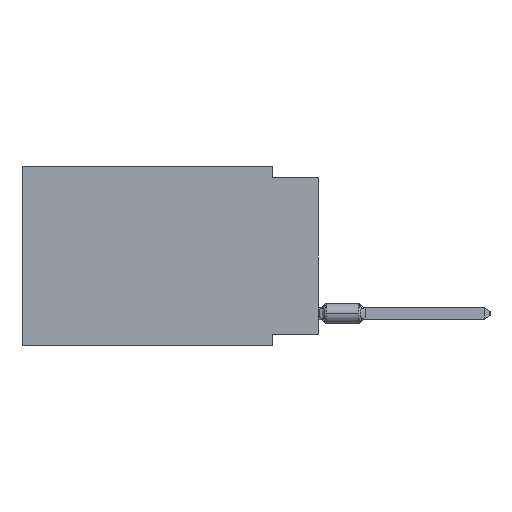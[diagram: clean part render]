
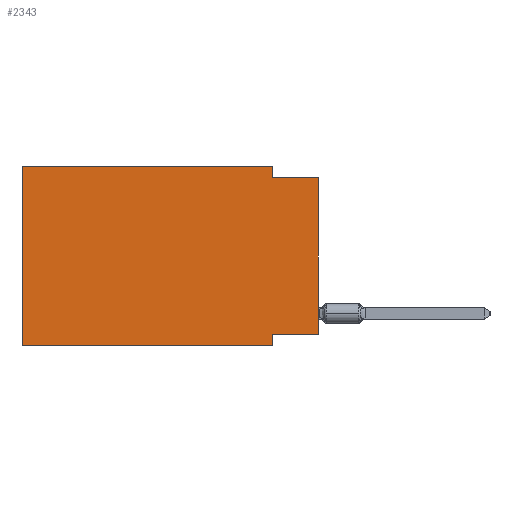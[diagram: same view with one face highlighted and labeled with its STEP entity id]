
A CAD part, left-side view. The second image highlights one B-rep face of the part: STEP entity #2343.
In plain terms, the highlighted planar face has unit normal (-1, 0, 0).
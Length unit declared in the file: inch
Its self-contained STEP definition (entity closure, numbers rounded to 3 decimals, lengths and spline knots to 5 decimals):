
#295 = CARTESIAN_POINT ( 'NONE',  ( 0., 0.1, 0. ) ) ;
#1831 = VERTEX_POINT ( 'NONE', #42576 ) ;
#2343 = ADVANCED_FACE ( 'NONE', ( #56258 ), #56657, .F. ) ;
#2878 = ORIENTED_EDGE ( 'NONE', *, *, #41714, .T. ) ;
#3446 = CARTESIAN_POINT ( 'NONE',  ( 0., 0., -0.365 ) ) ;
#5148 = EDGE_CURVE ( 'NONE', #18908, #56763, #9404, .T. ) ;
#6393 = ORIENTED_EDGE ( 'NONE', *, *, #54223, .F. ) ;
#6883 = CARTESIAN_POINT ( 'NONE',  ( 0., 0.645, -0.39 ) ) ;
#7452 = VECTOR ( 'NONE', #70423, 39.37008 ) ;
#9050 = DIRECTION ( 'NONE',  ( 0., -1., 0. ) ) ;
#9404 = LINE ( 'NONE', #3446, #15273 ) ;
#11210 = AXIS2_PLACEMENT_3D ( 'NONE', #44334, #33599, #42868 ) ;
#14451 = VECTOR ( 'NONE', #18934, 39.37008 ) ;
#14632 = CARTESIAN_POINT ( 'NONE',  ( 0., 0.645, -0.39 ) ) ;
#14707 = VERTEX_POINT ( 'NONE', #36645 ) ;
#15273 = VECTOR ( 'NONE', #33248, 39.37008 ) ;
#15733 = CARTESIAN_POINT ( 'NONE',  ( 0., 0.1, -0.39 ) ) ;
#15773 = VECTOR ( 'NONE', #32447, 39.37008 ) ;
#16245 = EDGE_LOOP ( 'NONE', ( #2878, #70546, #6393, #47762, #32399, #53599, #58178, #52525 ) ) ;
#17879 = CARTESIAN_POINT ( 'NONE',  ( 0., 0., -0.365 ) ) ;
#18908 = VERTEX_POINT ( 'NONE', #17879 ) ;
#18934 = DIRECTION ( 'NONE',  ( 0., -1., 0. ) ) ;
#19478 = DIRECTION ( 'NONE',  ( 0., 0., -1. ) ) ;
#19893 = VERTEX_POINT ( 'NONE', #75076 ) ;
#22936 = EDGE_CURVE ( 'NONE', #56229, #1831, #36547, .T. ) ;
#23877 = CARTESIAN_POINT ( 'NONE',  ( 0., 0.1, -0.365 ) ) ;
#25411 = CARTESIAN_POINT ( 'NONE',  ( 0., 0., -0.025 ) ) ;
#26595 = EDGE_CURVE ( 'NONE', #56763, #69303, #32579, .T. ) ;
#31820 = VECTOR ( 'NONE', #19478, 39.37008 ) ;
#32399 = ORIENTED_EDGE ( 'NONE', *, *, #22936, .F. ) ;
#32447 = DIRECTION ( 'NONE',  ( 0., 0., 1. ) ) ;
#32579 = LINE ( 'NONE', #67935, #31820 ) ;
#32872 = EDGE_CURVE ( 'NONE', #19893, #53914, #74124, .T. ) ;
#33248 = DIRECTION ( 'NONE',  ( 0., 1., 0. ) ) ;
#33599 = DIRECTION ( 'NONE',  ( 1., 0., 0. ) ) ;
#35204 = EDGE_CURVE ( 'NONE', #56229, #69303, #75773, .T. ) ;
#36071 = LINE ( 'NONE', #295, #45172 ) ;
#36547 = LINE ( 'NONE', #74522, #15773 ) ;
#36645 = CARTESIAN_POINT ( 'NONE',  ( 0., 0.1, 0. ) ) ;
#37546 = VECTOR ( 'NONE', #9050, 39.37008 ) ;
#39844 = LINE ( 'NONE', #57748, #7452 ) ;
#41714 = EDGE_CURVE ( 'NONE', #18908, #53914, #39844, .T. ) ;
#42576 = CARTESIAN_POINT ( 'NONE',  ( 0., 0.645, 0. ) ) ;
#42868 = DIRECTION ( 'NONE',  ( 0., 0., -1. ) ) ;
#44334 = CARTESIAN_POINT ( 'NONE',  ( 0., 0.645, 0. ) ) ;
#45172 = VECTOR ( 'NONE', #73755, 39.37008 ) ;
#47762 = ORIENTED_EDGE ( 'NONE', *, *, #77484, .F. ) ;
#50329 = CARTESIAN_POINT ( 'NONE',  ( 0., 0., -0.025 ) ) ;
#51799 = LINE ( 'NONE', #76793, #64509 ) ;
#52525 = ORIENTED_EDGE ( 'NONE', *, *, #5148, .F. ) ;
#52991 = DIRECTION ( 'NONE',  ( 0., -1., 0. ) ) ;
#53599 = ORIENTED_EDGE ( 'NONE', *, *, #35204, .T. ) ;
#53914 = VERTEX_POINT ( 'NONE', #25411 ) ;
#54223 = EDGE_CURVE ( 'NONE', #14707, #19893, #36071, .T. ) ;
#56229 = VERTEX_POINT ( 'NONE', #6883 ) ;
#56258 = FACE_OUTER_BOUND ( 'NONE', #16245, .T. ) ;
#56657 = PLANE ( 'NONE',  #11210 ) ;
#56763 = VERTEX_POINT ( 'NONE', #23877 ) ;
#57748 = CARTESIAN_POINT ( 'NONE',  ( 0., 0., 0. ) ) ;
#58178 = ORIENTED_EDGE ( 'NONE', *, *, #26595, .F. ) ;
#64509 = VECTOR ( 'NONE', #52991, 39.37008 ) ;
#67935 = CARTESIAN_POINT ( 'NONE',  ( 0., 0.1, -0.39 ) ) ;
#69303 = VERTEX_POINT ( 'NONE', #15733 ) ;
#70423 = DIRECTION ( 'NONE',  ( 0., 0., 1. ) ) ;
#70546 = ORIENTED_EDGE ( 'NONE', *, *, #32872, .F. ) ;
#73755 = DIRECTION ( 'NONE',  ( 0., 0., -1. ) ) ;
#74124 = LINE ( 'NONE', #50329, #14451 ) ;
#74522 = CARTESIAN_POINT ( 'NONE',  ( 0., 0.645, 0. ) ) ;
#75076 = CARTESIAN_POINT ( 'NONE',  ( 0., 0.1, -0.025 ) ) ;
#75773 = LINE ( 'NONE', #14632, #37546 ) ;
#76793 = CARTESIAN_POINT ( 'NONE',  ( 0., 0.645, 0. ) ) ;
#77484 = EDGE_CURVE ( 'NONE', #1831, #14707, #51799, .T. ) ;
